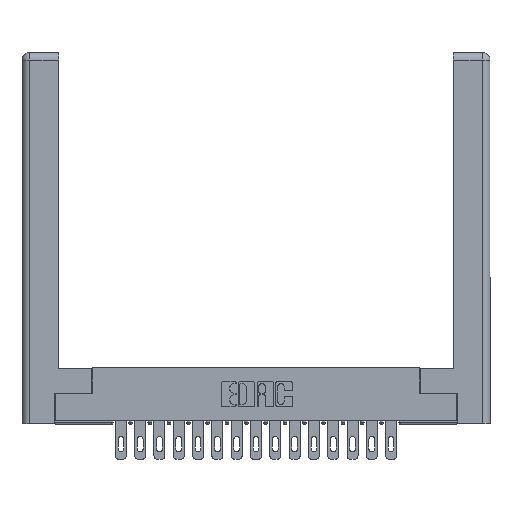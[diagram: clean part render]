
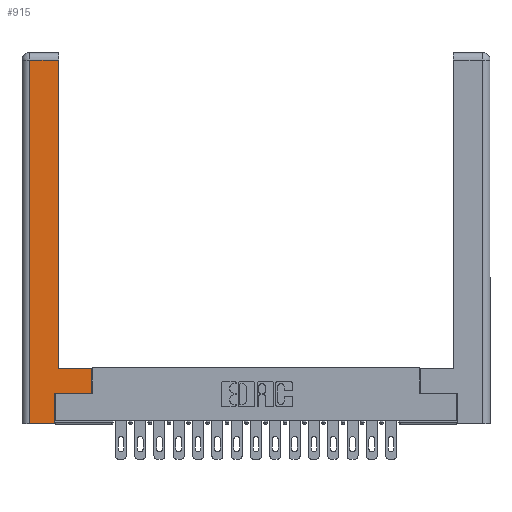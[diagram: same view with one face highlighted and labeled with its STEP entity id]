
A CAD part, top view. The second image highlights one B-rep face of the part: STEP entity #915.
In plain terms, the highlighted planar face has unit normal (0, 0, 1).
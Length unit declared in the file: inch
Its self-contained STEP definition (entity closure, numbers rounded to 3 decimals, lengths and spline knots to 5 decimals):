
#64 = VERTEX_POINT ( 'NONE', #2963 ) ;
#82 = DIRECTION ( 'NONE',  ( 0., 1., 0. ) ) ;
#125 = LINE ( 'NONE', #20224, #19719 ) ;
#303 = ORIENTED_EDGE ( 'NONE', *, *, #9448, .T. ) ;
#352 = DIRECTION ( 'NONE',  ( -1., 0., 0. ) ) ;
#646 = VERTEX_POINT ( 'NONE', #17866 ) ;
#817 = EDGE_CURVE ( 'NONE', #64, #6439, #14835, .T. ) ;
#915 = ADVANCED_FACE ( 'NONE', ( #6755 ), #1964, .F. ) ;
#1620 = VECTOR ( 'NONE', #4806, 39.37008 ) ;
#1964 = PLANE ( 'NONE',  #7745 ) ;
#2096 = CARTESIAN_POINT ( 'NONE',  ( 0.565, 0.245, 0. ) ) ;
#2273 = EDGE_CURVE ( 'NONE', #6439, #20100, #18400, .T. ) ;
#2490 = VECTOR ( 'NONE', #82, 39.37008 ) ;
#2624 = ORIENTED_EDGE ( 'NONE', *, *, #10369, .T. ) ;
#2963 = CARTESIAN_POINT ( 'NONE',  ( 0.265, 0., 0. ) ) ;
#3091 = VECTOR ( 'NONE', #352, 39.37008 ) ;
#3095 = CARTESIAN_POINT ( 'NONE',  ( 0.0615, 0., 0. ) ) ;
#3622 = LINE ( 'NONE', #19228, #3091 ) ;
#3658 = DIRECTION ( 'NONE',  ( 1., 0., 0. ) ) ;
#3768 = CARTESIAN_POINT ( 'NONE',  ( 0.295, 3., 0. ) ) ;
#4181 = VECTOR ( 'NONE', #3658, 39.37008 ) ;
#4806 = DIRECTION ( 'NONE',  ( 0., 1., 0. ) ) ;
#4959 = DIRECTION ( 'NONE',  ( -1., 0., 0. ) ) ;
#5384 = ORIENTED_EDGE ( 'NONE', *, *, #11726, .T. ) ;
#5721 = VECTOR ( 'NONE', #6950, 39.37008 ) ;
#6439 = VERTEX_POINT ( 'NONE', #10953 ) ;
#6755 = FACE_OUTER_BOUND ( 'NONE', #20046, .T. ) ;
#6950 = DIRECTION ( 'NONE',  ( 1., 0., 0. ) ) ;
#7160 = CARTESIAN_POINT ( 'NONE',  ( 0.265, 0.245, 0. ) ) ;
#7534 = CARTESIAN_POINT ( 'NONE',  ( 0.0615, 2.94, 0. ) ) ;
#7745 = AXIS2_PLACEMENT_3D ( 'NONE', #18697, #22089, #4959 ) ;
#7750 = DIRECTION ( 'NONE',  ( -1., 0., 0. ) ) ;
#8016 = ORIENTED_EDGE ( 'NONE', *, *, #19213, .T. ) ;
#8113 = VERTEX_POINT ( 'NONE', #10578 ) ;
#8352 = ORIENTED_EDGE ( 'NONE', *, *, #14655, .T. ) ;
#8374 = DIRECTION ( 'NONE',  ( 0., -1., 0. ) ) ;
#8557 = CARTESIAN_POINT ( 'NONE',  ( 0.295, 0.45, 0. ) ) ;
#8670 = EDGE_CURVE ( 'NONE', #14076, #8113, #11954, .T. ) ;
#9448 = EDGE_CURVE ( 'NONE', #16459, #14076, #3622, .T. ) ;
#9840 = VERTEX_POINT ( 'NONE', #3095 ) ;
#10369 = EDGE_CURVE ( 'NONE', #8113, #646, #12149, .T. ) ;
#10498 = ORIENTED_EDGE ( 'NONE', *, *, #817, .T. ) ;
#10556 = VECTOR ( 'NONE', #7750, 39.37008 ) ;
#10578 = CARTESIAN_POINT ( 'NONE',  ( 0.295, 2.94, 0. ) ) ;
#10831 = DIRECTION ( 'NONE',  ( 0., 1., 0. ) ) ;
#10953 = CARTESIAN_POINT ( 'NONE',  ( 0.265, 0.245, 0. ) ) ;
#11215 = CARTESIAN_POINT ( 'NONE',  ( 0.565, 0.245, 0. ) ) ;
#11726 = EDGE_CURVE ( 'NONE', #20100, #16459, #14795, .T. ) ;
#11954 = LINE ( 'NONE', #3768, #19239 ) ;
#12149 = LINE ( 'NONE', #7534, #10556 ) ;
#12884 = ORIENTED_EDGE ( 'NONE', *, *, #8670, .T. ) ;
#14027 = LINE ( 'NONE', #22188, #5721 ) ;
#14076 = VERTEX_POINT ( 'NONE', #8557 ) ;
#14655 = EDGE_CURVE ( 'NONE', #646, #9840, #125, .T. ) ;
#14795 = LINE ( 'NONE', #21938, #1620 ) ;
#14835 = LINE ( 'NONE', #7160, #2490 ) ;
#16459 = VERTEX_POINT ( 'NONE', #18418 ) ;
#17866 = CARTESIAN_POINT ( 'NONE',  ( 0.0615, 2.94, 0. ) ) ;
#18197 = ORIENTED_EDGE ( 'NONE', *, *, #2273, .T. ) ;
#18400 = LINE ( 'NONE', #2096, #4181 ) ;
#18418 = CARTESIAN_POINT ( 'NONE',  ( 0.565, 0.45, 0. ) ) ;
#18697 = CARTESIAN_POINT ( 'NONE',  ( 0., 0., 0. ) ) ;
#19213 = EDGE_CURVE ( 'NONE', #9840, #64, #14027, .T. ) ;
#19228 = CARTESIAN_POINT ( 'NONE',  ( 0.295, 0.45, 0. ) ) ;
#19239 = VECTOR ( 'NONE', #10831, 39.37008 ) ;
#19719 = VECTOR ( 'NONE', #8374, 39.37008 ) ;
#20046 = EDGE_LOOP ( 'NONE', ( #12884, #2624, #8352, #8016, #10498, #18197, #5384, #303 ) ) ;
#20100 = VERTEX_POINT ( 'NONE', #11215 ) ;
#20224 = CARTESIAN_POINT ( 'NONE',  ( 0.0615, 0., 0. ) ) ;
#21938 = CARTESIAN_POINT ( 'NONE',  ( 0.565, 0.45, 0. ) ) ;
#22089 = DIRECTION ( 'NONE',  ( 0., 0., -1. ) ) ;
#22188 = CARTESIAN_POINT ( 'NONE',  ( 0.265, 0., 0. ) ) ;
